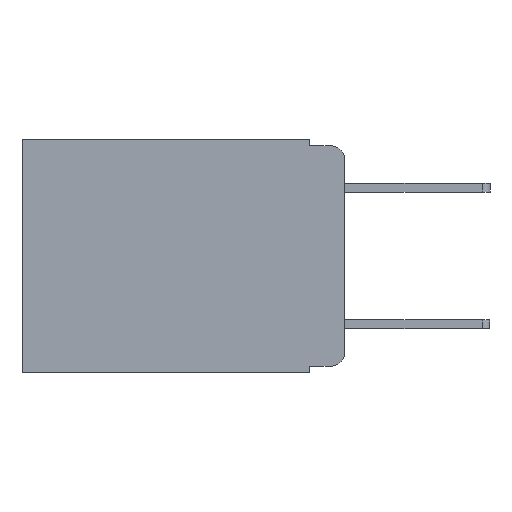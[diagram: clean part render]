
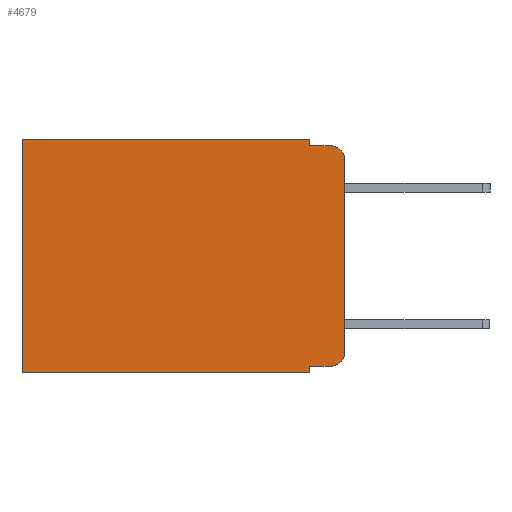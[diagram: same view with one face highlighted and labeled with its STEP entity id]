
A CAD part, left-side view. The second image highlights one B-rep face of the part: STEP entity #4679.
In plain terms, the highlighted planar face has unit normal (-1, 0, 0).
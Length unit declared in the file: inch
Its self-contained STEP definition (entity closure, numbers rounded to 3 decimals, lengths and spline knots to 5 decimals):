
#27 = VECTOR ( 'NONE', #2352, 39.37008 ) ;
#70 = DIRECTION ( 'NONE',  ( -1., 0., 0. ) ) ;
#282 = DIRECTION ( 'NONE',  ( 0., 0., -1. ) ) ;
#311 = CARTESIAN_POINT ( 'NONE',  ( 0.298, 0., 0. ) ) ;
#319 = CARTESIAN_POINT ( 'NONE',  ( 0.298, 0., 0. ) ) ;
#540 = EDGE_CURVE ( 'NONE', #4293, #8130, #8634, .T. ) ;
#810 = DIRECTION ( 'NONE',  ( 0., -1., 0. ) ) ;
#828 = LINE ( 'NONE', #3705, #5264 ) ;
#952 = CARTESIAN_POINT ( 'NONE',  ( 0.298, 0.02, -0.333 ) ) ;
#1048 = ORIENTED_EDGE ( 'NONE', *, *, #2799, .F. ) ;
#1061 = EDGE_LOOP ( 'NONE', ( #3338, #9585, #5638, #6140, #2092, #5491, #1382, #1048, #1186, #2770 ) ) ;
#1062 = AXIS2_PLACEMENT_3D ( 'NONE', #8070, #6129, #282 ) ;
#1167 = VERTEX_POINT ( 'NONE', #3074 ) ;
#1186 = ORIENTED_EDGE ( 'NONE', *, *, #7265, .T. ) ;
#1237 = CARTESIAN_POINT ( 'NONE',  ( 0.298, 0.02, -0.313 ) ) ;
#1251 = VECTOR ( 'NONE', #9242, 39.37008 ) ;
#1349 = CARTESIAN_POINT ( 'NONE',  ( 0.298, 0.02, -0.01 ) ) ;
#1382 = ORIENTED_EDGE ( 'NONE', *, *, #7112, .F. ) ;
#1461 = CARTESIAN_POINT ( 'NONE',  ( 0.298, 0.473, 0. ) ) ;
#1519 = CARTESIAN_POINT ( 'NONE',  ( 0.298, 0., -0.03 ) ) ;
#1559 = CARTESIAN_POINT ( 'NONE',  ( 0.298, 0.051, -0.343 ) ) ;
#1591 = LINE ( 'NONE', #1461, #10139 ) ;
#1934 = EDGE_CURVE ( 'NONE', #4426, #6085, #828, .T. ) ;
#2092 = ORIENTED_EDGE ( 'NONE', *, *, #3863, .T. ) ;
#2352 = DIRECTION ( 'NONE',  ( 0., 1., 0. ) ) ;
#2560 = VECTOR ( 'NONE', #8232, 39.37008 ) ;
#2667 = DIRECTION ( 'NONE',  ( 0., 0., -1. ) ) ;
#2678 = DIRECTION ( 'NONE',  ( -1., 0., 0. ) ) ;
#2770 = ORIENTED_EDGE ( 'NONE', *, *, #3036, .T. ) ;
#2799 = EDGE_CURVE ( 'NONE', #8667, #7179, #5894, .T. ) ;
#2963 = AXIS2_PLACEMENT_3D ( 'NONE', #5357, #70, #6159 ) ;
#3036 = EDGE_CURVE ( 'NONE', #6073, #8130, #3232, .T. ) ;
#3074 = CARTESIAN_POINT ( 'NONE',  ( 0.298, 0.473, 0. ) ) ;
#3192 = FACE_OUTER_BOUND ( 'NONE', #1061, .T. ) ;
#3232 = CIRCLE ( 'NONE', #5199, 0.02 ) ;
#3338 = ORIENTED_EDGE ( 'NONE', *, *, #540, .F. ) ;
#3566 = LINE ( 'NONE', #7612, #5802 ) ;
#3705 = CARTESIAN_POINT ( 'NONE',  ( 0.298, 0.051, 0. ) ) ;
#3710 = DIRECTION ( 'NONE',  ( 0., 0., -1. ) ) ;
#3863 = EDGE_CURVE ( 'NONE', #4426, #1167, #10765, .T. ) ;
#4145 = DIRECTION ( 'NONE',  ( 0., -1., 0. ) ) ;
#4293 = VERTEX_POINT ( 'NONE', #1519 ) ;
#4426 = VERTEX_POINT ( 'NONE', #8761 ) ;
#4679 = ADVANCED_FACE ( 'NONE', ( #3192 ), #5254, .F. ) ;
#4900 = CIRCLE ( 'NONE', #2963, 0.02 ) ;
#5199 = AXIS2_PLACEMENT_3D ( 'NONE', #1237, #2678, #2667 ) ;
#5254 = PLANE ( 'NONE',  #1062 ) ;
#5264 = VECTOR ( 'NONE', #3710, 39.37008 ) ;
#5357 = CARTESIAN_POINT ( 'NONE',  ( 0.298, 0.02, -0.03 ) ) ;
#5469 = EDGE_CURVE ( 'NONE', #1167, #6483, #1591, .T. ) ;
#5491 = ORIENTED_EDGE ( 'NONE', *, *, #5469, .T. ) ;
#5638 = ORIENTED_EDGE ( 'NONE', *, *, #7070, .F. ) ;
#5802 = VECTOR ( 'NONE', #810, 39.37008 ) ;
#5894 = LINE ( 'NONE', #9380, #1251 ) ;
#6073 = VERTEX_POINT ( 'NONE', #952 ) ;
#6085 = VERTEX_POINT ( 'NONE', #8538 ) ;
#6129 = DIRECTION ( 'NONE',  ( 1., 0., 0. ) ) ;
#6140 = ORIENTED_EDGE ( 'NONE', *, *, #1934, .F. ) ;
#6159 = DIRECTION ( 'NONE',  ( 0., 0., -1. ) ) ;
#6483 = VERTEX_POINT ( 'NONE', #10506 ) ;
#6618 = VECTOR ( 'NONE', #10456, 39.37008 ) ;
#6900 = LINE ( 'NONE', #9004, #27 ) ;
#6917 = CARTESIAN_POINT ( 'NONE',  ( 0.298, 0., -0.313 ) ) ;
#7070 = EDGE_CURVE ( 'NONE', #6085, #8465, #9246, .T. ) ;
#7112 = EDGE_CURVE ( 'NONE', #7179, #6483, #6900, .T. ) ;
#7141 = VECTOR ( 'NONE', #4145, 39.37008 ) ;
#7179 = VERTEX_POINT ( 'NONE', #1559 ) ;
#7265 = EDGE_CURVE ( 'NONE', #8667, #6073, #3566, .T. ) ;
#7349 = CARTESIAN_POINT ( 'NONE',  ( 0.298, 0.051, -0.01 ) ) ;
#7612 = CARTESIAN_POINT ( 'NONE',  ( 0.298, 0.051, -0.333 ) ) ;
#8070 = CARTESIAN_POINT ( 'NONE',  ( 0.298, 0., 0. ) ) ;
#8130 = VERTEX_POINT ( 'NONE', #6917 ) ;
#8134 = EDGE_CURVE ( 'NONE', #4293, #8465, #4900, .T. ) ;
#8232 = DIRECTION ( 'NONE',  ( 0., 0., -1. ) ) ;
#8465 = VERTEX_POINT ( 'NONE', #1349 ) ;
#8538 = CARTESIAN_POINT ( 'NONE',  ( 0.298, 0.051, -0.01 ) ) ;
#8634 = LINE ( 'NONE', #311, #2560 ) ;
#8667 = VERTEX_POINT ( 'NONE', #9087 ) ;
#8761 = CARTESIAN_POINT ( 'NONE',  ( 0.298, 0.051, 0. ) ) ;
#9004 = CARTESIAN_POINT ( 'NONE',  ( 0.298, 0., -0.343 ) ) ;
#9087 = CARTESIAN_POINT ( 'NONE',  ( 0.298, 0.051, -0.333 ) ) ;
#9242 = DIRECTION ( 'NONE',  ( 0., 0., -1. ) ) ;
#9246 = LINE ( 'NONE', #7349, #7141 ) ;
#9380 = CARTESIAN_POINT ( 'NONE',  ( 0.298, 0.051, 0. ) ) ;
#9478 = DIRECTION ( 'NONE',  ( 0., 0., -1. ) ) ;
#9585 = ORIENTED_EDGE ( 'NONE', *, *, #8134, .T. ) ;
#10139 = VECTOR ( 'NONE', #9478, 39.37008 ) ;
#10456 = DIRECTION ( 'NONE',  ( 0., 1., 0. ) ) ;
#10506 = CARTESIAN_POINT ( 'NONE',  ( 0.298, 0.473, -0.343 ) ) ;
#10765 = LINE ( 'NONE', #319, #6618 ) ;
